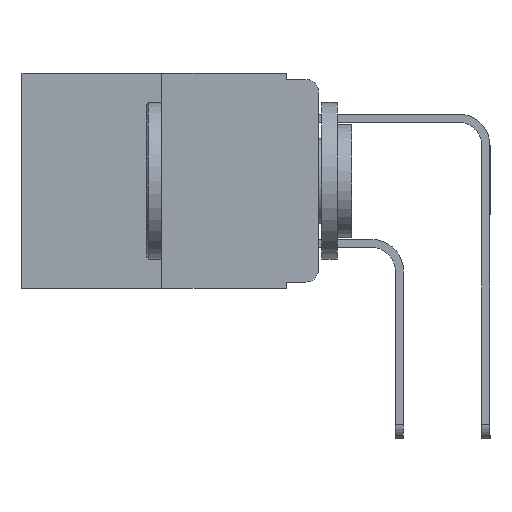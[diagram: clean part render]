
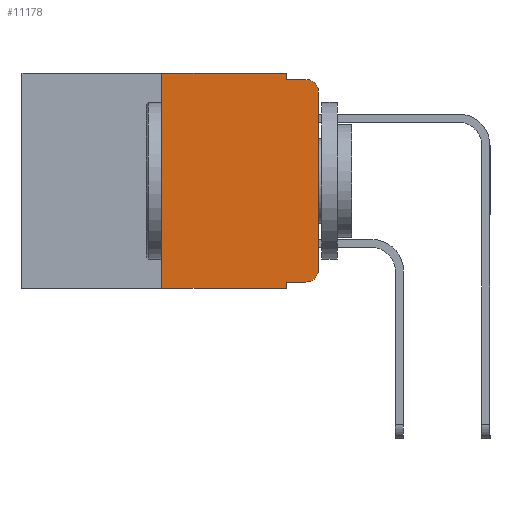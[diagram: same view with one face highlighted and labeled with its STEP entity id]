
A CAD part, left-side view. The second image highlights one B-rep face of the part: STEP entity #11178.
In plain terms, the highlighted planar face has unit normal (-1, 0, 0).
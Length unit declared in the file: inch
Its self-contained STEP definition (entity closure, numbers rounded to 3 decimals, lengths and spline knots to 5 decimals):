
#272 = VECTOR ( 'NONE', #5651, 39.37008 ) ;
#353 = EDGE_CURVE ( 'NONE', #13146, #3619, #3752, .T. ) ;
#511 = VERTEX_POINT ( 'NONE', #5561 ) ;
#1628 = CARTESIAN_POINT ( 'NONE',  ( 0., 0.051, 0. ) ) ;
#1644 = VECTOR ( 'NONE', #6719, 39.37008 ) ;
#1900 = DIRECTION ( 'NONE',  ( -1., 0., 0. ) ) ;
#2136 = CARTESIAN_POINT ( 'NONE',  ( 0., 0.051, -0.333 ) ) ;
#2381 = VECTOR ( 'NONE', #3217, 39.37008 ) ;
#2661 = CARTESIAN_POINT ( 'NONE',  ( 0., 0.051, 0. ) ) ;
#2692 = ORIENTED_EDGE ( 'NONE', *, *, #10106, .T. ) ;
#3001 = FACE_OUTER_BOUND ( 'NONE', #7674, .T. ) ;
#3009 = CARTESIAN_POINT ( 'NONE',  ( 0., 0., 0. ) ) ;
#3061 = DIRECTION ( 'NONE',  ( 0., 0., 1. ) ) ;
#3217 = DIRECTION ( 'NONE',  ( 0., 0., 1. ) ) ;
#3285 = LINE ( 'NONE', #7958, #11379 ) ;
#3446 = EDGE_CURVE ( 'NONE', #8058, #13329, #12939, .T. ) ;
#3619 = VERTEX_POINT ( 'NONE', #7031 ) ;
#3752 = LINE ( 'NONE', #2661, #7026 ) ;
#3953 = LINE ( 'NONE', #10644, #6555 ) ;
#4508 = CARTESIAN_POINT ( 'NONE',  ( 0., 0.473, -0.343 ) ) ;
#4587 = EDGE_CURVE ( 'NONE', #11798, #3619, #7973, .T. ) ;
#4619 = VERTEX_POINT ( 'NONE', #10033 ) ;
#4794 = VECTOR ( 'NONE', #3061, 39.37008 ) ;
#4987 = PLANE ( 'NONE',  #14365 ) ;
#5032 = EDGE_CURVE ( 'NONE', #11798, #4619, #10871, .T. ) ;
#5221 = EDGE_CURVE ( 'NONE', #5740, #13329, #3285, .T. ) ;
#5561 = CARTESIAN_POINT ( 'NONE',  ( 0., 0., -0.313 ) ) ;
#5651 = DIRECTION ( 'NONE',  ( 0., -1., 0. ) ) ;
#5740 = VERTEX_POINT ( 'NONE', #9957 ) ;
#6040 = CARTESIAN_POINT ( 'NONE',  ( 0., 0.25, -0.343 ) ) ;
#6555 = VECTOR ( 'NONE', #7390, 39.37008 ) ;
#6719 = DIRECTION ( 'NONE',  ( 0., -1., 0. ) ) ;
#6757 = CARTESIAN_POINT ( 'NONE',  ( 0., 0.051, -0.333 ) ) ;
#7026 = VECTOR ( 'NONE', #7194, 39.37008 ) ;
#7031 = CARTESIAN_POINT ( 'NONE',  ( 0., 0.051, -0.343 ) ) ;
#7194 = DIRECTION ( 'NONE',  ( 0., 0., -1. ) ) ;
#7215 = DIRECTION ( 'NONE',  ( 0., 0., -1. ) ) ;
#7390 = DIRECTION ( 'NONE',  ( 0., -1., 0. ) ) ;
#7652 = ORIENTED_EDGE ( 'NONE', *, *, #5221, .F. ) ;
#7674 = EDGE_LOOP ( 'NONE', ( #2692, #7779, #7652, #13121, #10576, #11570, #8829, #9843, #10114, #9395 ) ) ;
#7779 = ORIENTED_EDGE ( 'NONE', *, *, #3446, .T. ) ;
#7958 = CARTESIAN_POINT ( 'NONE',  ( 0., 0.051, -0.01 ) ) ;
#7973 = LINE ( 'NONE', #4508, #1644 ) ;
#8058 = VERTEX_POINT ( 'NONE', #9740 ) ;
#8068 = LINE ( 'NONE', #3009, #4794 ) ;
#8174 = VERTEX_POINT ( 'NONE', #10982 ) ;
#8262 = EDGE_CURVE ( 'NONE', #13146, #8174, #9309, .T. ) ;
#8352 = AXIS2_PLACEMENT_3D ( 'NONE', #8611, #1900, #9700 ) ;
#8363 = DIRECTION ( 'NONE',  ( 0., 0., -1. ) ) ;
#8611 = CARTESIAN_POINT ( 'NONE',  ( 0., 0.02, -0.313 ) ) ;
#8746 = CARTESIAN_POINT ( 'NONE',  ( 0., 0.25, 0. ) ) ;
#8829 = ORIENTED_EDGE ( 'NONE', *, *, #4587, .T. ) ;
#8840 = AXIS2_PLACEMENT_3D ( 'NONE', #9976, #9942, #11411 ) ;
#9309 = LINE ( 'NONE', #6757, #272 ) ;
#9395 = ORIENTED_EDGE ( 'NONE', *, *, #11358, .T. ) ;
#9412 = CIRCLE ( 'NONE', #8352, 0.02 ) ;
#9700 = DIRECTION ( 'NONE',  ( 0., 0., -1. ) ) ;
#9740 = CARTESIAN_POINT ( 'NONE',  ( 0., 0., -0.03 ) ) ;
#9843 = ORIENTED_EDGE ( 'NONE', *, *, #353, .F. ) ;
#9917 = EDGE_CURVE ( 'NONE', #10182, #5740, #13323, .T. ) ;
#9942 = DIRECTION ( 'NONE',  ( -1., 0., 0. ) ) ;
#9957 = CARTESIAN_POINT ( 'NONE',  ( 0., 0.051, -0.01 ) ) ;
#9976 = CARTESIAN_POINT ( 'NONE',  ( 0., 0.02, -0.03 ) ) ;
#10033 = CARTESIAN_POINT ( 'NONE',  ( 0., 0.25, 0. ) ) ;
#10106 = EDGE_CURVE ( 'NONE', #511, #8058, #8068, .T. ) ;
#10114 = ORIENTED_EDGE ( 'NONE', *, *, #8262, .T. ) ;
#10182 = VERTEX_POINT ( 'NONE', #14255 ) ;
#10291 = CARTESIAN_POINT ( 'NONE',  ( 0., 0.02, -0.01 ) ) ;
#10576 = ORIENTED_EDGE ( 'NONE', *, *, #14193, .F. ) ;
#10644 = CARTESIAN_POINT ( 'NONE',  ( 0., 0.473, 0. ) ) ;
#10871 = LINE ( 'NONE', #8746, #2381 ) ;
#10982 = CARTESIAN_POINT ( 'NONE',  ( 0., 0.02, -0.333 ) ) ;
#11178 = ADVANCED_FACE ( 'NONE', ( #3001 ), #4987, .F. ) ;
#11358 = EDGE_CURVE ( 'NONE', #8174, #511, #9412, .T. ) ;
#11379 = VECTOR ( 'NONE', #12320, 39.37008 ) ;
#11411 = DIRECTION ( 'NONE',  ( 0., 0., -1. ) ) ;
#11570 = ORIENTED_EDGE ( 'NONE', *, *, #5032, .F. ) ;
#11798 = VERTEX_POINT ( 'NONE', #6040 ) ;
#12320 = DIRECTION ( 'NONE',  ( 0., -1., 0. ) ) ;
#12650 = CARTESIAN_POINT ( 'NONE',  ( 0., 0.473, 0. ) ) ;
#12939 = CIRCLE ( 'NONE', #8840, 0.02 ) ;
#13004 = VECTOR ( 'NONE', #8363, 39.37008 ) ;
#13121 = ORIENTED_EDGE ( 'NONE', *, *, #9917, .F. ) ;
#13146 = VERTEX_POINT ( 'NONE', #2136 ) ;
#13323 = LINE ( 'NONE', #1628, #13004 ) ;
#13329 = VERTEX_POINT ( 'NONE', #10291 ) ;
#13682 = DIRECTION ( 'NONE',  ( 1., 0., 0. ) ) ;
#14193 = EDGE_CURVE ( 'NONE', #4619, #10182, #3953, .T. ) ;
#14255 = CARTESIAN_POINT ( 'NONE',  ( 0., 0.051, 0. ) ) ;
#14365 = AXIS2_PLACEMENT_3D ( 'NONE', #12650, #13682, #7215 ) ;
